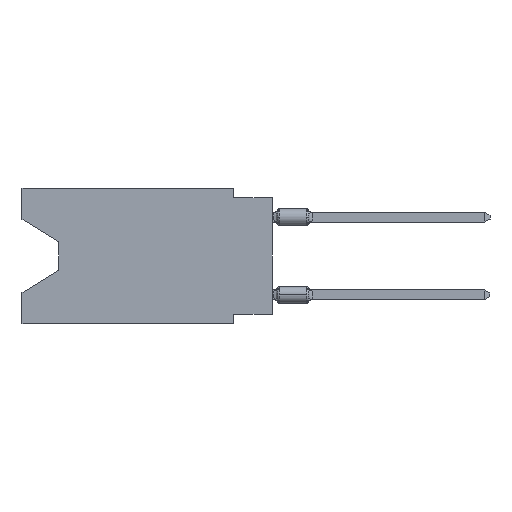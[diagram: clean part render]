
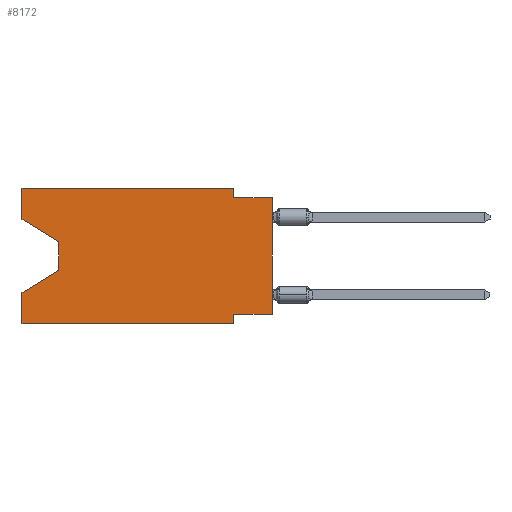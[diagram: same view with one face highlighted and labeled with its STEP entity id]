
A CAD part, left-side view. The second image highlights one B-rep face of the part: STEP entity #8172.
In plain terms, the highlighted planar face has unit normal (-1, 0, 0).
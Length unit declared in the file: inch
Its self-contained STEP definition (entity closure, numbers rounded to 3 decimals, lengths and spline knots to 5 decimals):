
#319 = EDGE_CURVE ( 'NONE', #8990, #32838, #5875, .T. ) ;
#1085 = LINE ( 'NONE', #26274, #6271 ) ;
#1675 = LINE ( 'NONE', #9974, #36947 ) ;
#1933 = ORIENTED_EDGE ( 'NONE', *, *, #14924, .F. ) ;
#3134 = CARTESIAN_POINT ( 'NONE',  ( 0., 0.55, -0.212 ) ) ;
#3956 = ORIENTED_EDGE ( 'NONE', *, *, #12091, .F. ) ;
#4036 = LINE ( 'NONE', #54674, #10957 ) ;
#5295 = CARTESIAN_POINT ( 'NONE',  ( 0., 0.645, -0.35 ) ) ;
#5424 = VECTOR ( 'NONE', #27413, 39.37008 ) ;
#5456 = VERTEX_POINT ( 'NONE', #14844 ) ;
#5875 = LINE ( 'NONE', #22748, #25802 ) ;
#6042 = VERTEX_POINT ( 'NONE', #54646 ) ;
#6271 = VECTOR ( 'NONE', #26546, 39.37008 ) ;
#7260 = FACE_OUTER_BOUND ( 'NONE', #49363, .T. ) ;
#8172 = ADVANCED_FACE ( 'NONE', ( #7260 ), #32708, .F. ) ;
#8203 = CARTESIAN_POINT ( 'NONE',  ( 0., 0.1, 0. ) ) ;
#8990 = VERTEX_POINT ( 'NONE', #25516 ) ;
#9892 = VERTEX_POINT ( 'NONE', #50556 ) ;
#9974 = CARTESIAN_POINT ( 'NONE',  ( 0., 0.645, 0. ) ) ;
#10139 = VECTOR ( 'NONE', #21142, 39.37008 ) ;
#10544 = CARTESIAN_POINT ( 'NONE',  ( 0., 0.645, -0.08025 ) ) ;
#10957 = VECTOR ( 'NONE', #37772, 39.37008 ) ;
#12091 = EDGE_CURVE ( 'NONE', #15214, #32838, #25729, .T. ) ;
#12756 = VECTOR ( 'NONE', #34597, 39.37008 ) ;
#13217 = EDGE_CURVE ( 'NONE', #13542, #6042, #31296, .T. ) ;
#13542 = VERTEX_POINT ( 'NONE', #43677 ) ;
#14629 = CARTESIAN_POINT ( 'NONE',  ( 0., 0.645, 0. ) ) ;
#14844 = CARTESIAN_POINT ( 'NONE',  ( 0., 0.1, -0.325 ) ) ;
#14924 = EDGE_CURVE ( 'NONE', #37444, #34068, #23446, .T. ) ;
#15214 = VERTEX_POINT ( 'NONE', #21771 ) ;
#16143 = DIRECTION ( 'NONE',  ( 0., 0.855, -0.519 ) ) ;
#16613 = CARTESIAN_POINT ( 'NONE',  ( 0., 0., -0.025 ) ) ;
#16883 = DIRECTION ( 'NONE',  ( 0., -1., 0. ) ) ;
#17174 = VECTOR ( 'NONE', #42509, 39.37008 ) ;
#19422 = DIRECTION ( 'NONE',  ( 0., 0., -1. ) ) ;
#19448 = ORIENTED_EDGE ( 'NONE', *, *, #49884, .F. ) ;
#20287 = CARTESIAN_POINT ( 'NONE',  ( 0., 0.645, 0. ) ) ;
#20589 = LINE ( 'NONE', #29697, #10139 ) ;
#21142 = DIRECTION ( 'NONE',  ( 0., -1., 0. ) ) ;
#21615 = LINE ( 'NONE', #42362, #12756 ) ;
#21771 = CARTESIAN_POINT ( 'NONE',  ( 0., 0.1, -0.025 ) ) ;
#22748 = CARTESIAN_POINT ( 'NONE',  ( 0., 0., 0. ) ) ;
#23037 = ORIENTED_EDGE ( 'NONE', *, *, #32716, .T. ) ;
#23446 = LINE ( 'NONE', #14629, #51152 ) ;
#24570 = ORIENTED_EDGE ( 'NONE', *, *, #29777, .F. ) ;
#25516 = CARTESIAN_POINT ( 'NONE',  ( 0., 0., -0.325 ) ) ;
#25729 = LINE ( 'NONE', #16613, #49466 ) ;
#25802 = VECTOR ( 'NONE', #47920, 39.37008 ) ;
#25927 = ORIENTED_EDGE ( 'NONE', *, *, #13217, .T. ) ;
#26274 = CARTESIAN_POINT ( 'NONE',  ( 0., 0., -0.325 ) ) ;
#26546 = DIRECTION ( 'NONE',  ( 0., 1., 0. ) ) ;
#26572 = DIRECTION ( 'NONE',  ( 0., 0., 1. ) ) ;
#26800 = EDGE_CURVE ( 'NONE', #13542, #40781, #1675, .T. ) ;
#27413 = DIRECTION ( 'NONE',  ( 0., -0.855, -0.519 ) ) ;
#28118 = VERTEX_POINT ( 'NONE', #39084 ) ;
#28528 = LINE ( 'NONE', #49541, #42877 ) ;
#29613 = CARTESIAN_POINT ( 'NONE',  ( 0., 0., -0.025 ) ) ;
#29697 = CARTESIAN_POINT ( 'NONE',  ( 0., 0.645, 0. ) ) ;
#29777 = EDGE_CURVE ( 'NONE', #5456, #43146, #21615, .T. ) ;
#31127 = VECTOR ( 'NONE', #16143, 39.37008 ) ;
#31221 = EDGE_CURVE ( 'NONE', #37444, #43146, #4036, .T. ) ;
#31253 = CARTESIAN_POINT ( 'NONE',  ( 0., 0.645, -0.26975 ) ) ;
#31296 = LINE ( 'NONE', #10544, #5424 ) ;
#31655 = EDGE_CURVE ( 'NONE', #40781, #9892, #20589, .T. ) ;
#32708 = PLANE ( 'NONE',  #41967 ) ;
#32716 = EDGE_CURVE ( 'NONE', #6042, #28118, #28528, .T. ) ;
#32838 = VERTEX_POINT ( 'NONE', #29613 ) ;
#34068 = VERTEX_POINT ( 'NONE', #31253 ) ;
#34597 = DIRECTION ( 'NONE',  ( 0., 0., -1. ) ) ;
#36006 = ORIENTED_EDGE ( 'NONE', *, *, #53779, .F. ) ;
#36357 = ORIENTED_EDGE ( 'NONE', *, *, #31221, .T. ) ;
#36947 = VECTOR ( 'NONE', #26572, 39.37008 ) ;
#36981 = CARTESIAN_POINT ( 'NONE',  ( 0., 0.645, 0. ) ) ;
#37134 = DIRECTION ( 'NONE',  ( 1., 0., 0. ) ) ;
#37444 = VERTEX_POINT ( 'NONE', #5295 ) ;
#37772 = DIRECTION ( 'NONE',  ( 0., -1., 0. ) ) ;
#38497 = ORIENTED_EDGE ( 'NONE', *, *, #51027, .T. ) ;
#39084 = CARTESIAN_POINT ( 'NONE',  ( 0., 0.55, -0.212 ) ) ;
#40232 = ORIENTED_EDGE ( 'NONE', *, *, #319, .T. ) ;
#40781 = VERTEX_POINT ( 'NONE', #36981 ) ;
#41200 = ORIENTED_EDGE ( 'NONE', *, *, #26800, .F. ) ;
#41317 = LINE ( 'NONE', #3134, #31127 ) ;
#41967 = AXIS2_PLACEMENT_3D ( 'NONE', #20287, #37134, #49863 ) ;
#42362 = CARTESIAN_POINT ( 'NONE',  ( 0., 0.1, -0.35 ) ) ;
#42509 = DIRECTION ( 'NONE',  ( 0., 0., -1. ) ) ;
#42877 = VECTOR ( 'NONE', #19422, 39.37008 ) ;
#43146 = VERTEX_POINT ( 'NONE', #47118 ) ;
#43677 = CARTESIAN_POINT ( 'NONE',  ( 0., 0.645, -0.08025 ) ) ;
#44202 = DIRECTION ( 'NONE',  ( 0., 0., 1. ) ) ;
#44756 = ORIENTED_EDGE ( 'NONE', *, *, #31655, .F. ) ;
#47118 = CARTESIAN_POINT ( 'NONE',  ( 0., 0.1, -0.35 ) ) ;
#47920 = DIRECTION ( 'NONE',  ( 0., 0., 1. ) ) ;
#49363 = EDGE_LOOP ( 'NONE', ( #25927, #23037, #38497, #1933, #36357, #24570, #19448, #40232, #3956, #36006, #44756, #41200 ) ) ;
#49466 = VECTOR ( 'NONE', #16883, 39.37008 ) ;
#49541 = CARTESIAN_POINT ( 'NONE',  ( 0., 0.55, -0.138 ) ) ;
#49863 = DIRECTION ( 'NONE',  ( 0., 0., -1. ) ) ;
#49884 = EDGE_CURVE ( 'NONE', #8990, #5456, #1085, .T. ) ;
#50255 = LINE ( 'NONE', #8203, #17174 ) ;
#50556 = CARTESIAN_POINT ( 'NONE',  ( 0., 0.1, 0. ) ) ;
#51027 = EDGE_CURVE ( 'NONE', #28118, #34068, #41317, .T. ) ;
#51152 = VECTOR ( 'NONE', #44202, 39.37008 ) ;
#53779 = EDGE_CURVE ( 'NONE', #9892, #15214, #50255, .T. ) ;
#54646 = CARTESIAN_POINT ( 'NONE',  ( 0., 0.55, -0.138 ) ) ;
#54674 = CARTESIAN_POINT ( 'NONE',  ( 0., 0.645, -0.35 ) ) ;
